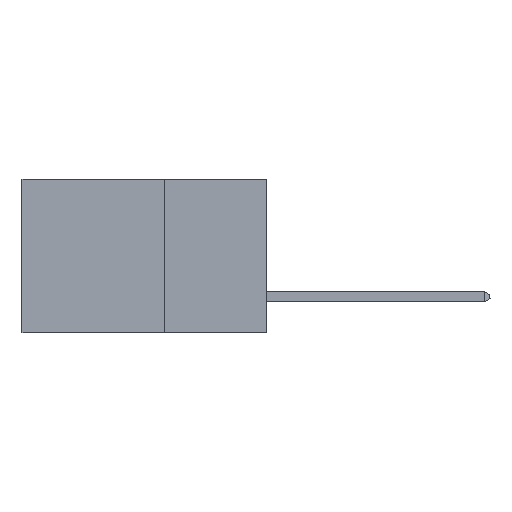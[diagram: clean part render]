
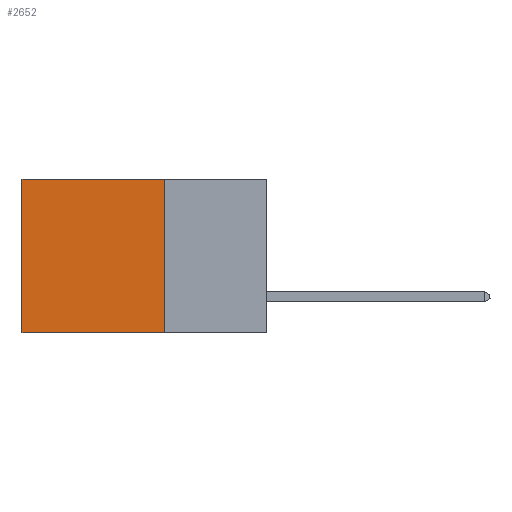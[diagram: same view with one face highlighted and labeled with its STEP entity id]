
A CAD part, left-side view. The second image highlights one B-rep face of the part: STEP entity #2652.
In plain terms, the highlighted planar face has unit normal (-1, 0, 0).
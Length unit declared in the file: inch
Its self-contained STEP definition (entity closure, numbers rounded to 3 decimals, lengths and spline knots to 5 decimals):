
#271 = CARTESIAN_POINT ( 'NONE',  ( 0.2875, 0.25, 0. ) ) ;
#722 = CARTESIAN_POINT ( 'NONE',  ( 0.2875, 0.25, -0.375 ) ) ;
#2652 = ADVANCED_FACE ( 'NONE', ( #4396 ), #6562, .F. ) ;
#2677 = VECTOR ( 'NONE', #5088, 39.37008 ) ;
#2813 = EDGE_CURVE ( 'NONE', #5606, #12103, #5889, .T. ) ;
#3095 = CARTESIAN_POINT ( 'NONE',  ( 0.2875, 0.25, -0.375 ) ) ;
#3446 = ORIENTED_EDGE ( 'NONE', *, *, #2813, .T. ) ;
#3755 = VECTOR ( 'NONE', #7795, 39.37008 ) ;
#3766 = ORIENTED_EDGE ( 'NONE', *, *, #13900, .F. ) ;
#4256 = CARTESIAN_POINT ( 'NONE',  ( 0.2875, 0.6, -0.375 ) ) ;
#4271 = VERTEX_POINT ( 'NONE', #7142 ) ;
#4396 = FACE_OUTER_BOUND ( 'NONE', #11799, .T. ) ;
#4600 = CARTESIAN_POINT ( 'NONE',  ( 0.2875, 0.25, -0.375 ) ) ;
#5088 = DIRECTION ( 'NONE',  ( 0., 1., 0. ) ) ;
#5606 = VERTEX_POINT ( 'NONE', #7146 ) ;
#5709 = LINE ( 'NONE', #12401, #6722 ) ;
#5889 = LINE ( 'NONE', #6635, #3755 ) ;
#5900 = LINE ( 'NONE', #4600, #6425 ) ;
#6425 = VECTOR ( 'NONE', #9101, 39.37008 ) ;
#6562 = PLANE ( 'NONE',  #11405 ) ;
#6635 = CARTESIAN_POINT ( 'NONE',  ( 0.2875, 0.6, -0.375 ) ) ;
#6722 = VECTOR ( 'NONE', #8974, 39.37008 ) ;
#6753 = EDGE_CURVE ( 'NONE', #11811, #5606, #5709, .T. ) ;
#7142 = CARTESIAN_POINT ( 'NONE',  ( 0.2875, 0.25, -0.375 ) ) ;
#7146 = CARTESIAN_POINT ( 'NONE',  ( 0.2875, 0.6, 0. ) ) ;
#7255 = LINE ( 'NONE', #722, #2677 ) ;
#7795 = DIRECTION ( 'NONE',  ( 0., 0., -1. ) ) ;
#8974 = DIRECTION ( 'NONE',  ( 0., 1., 0. ) ) ;
#9101 = DIRECTION ( 'NONE',  ( 0., 0., -1. ) ) ;
#9267 = EDGE_CURVE ( 'NONE', #4271, #12103, #7255, .T. ) ;
#9344 = ORIENTED_EDGE ( 'NONE', *, *, #9267, .F. ) ;
#11082 = ORIENTED_EDGE ( 'NONE', *, *, #6753, .T. ) ;
#11405 = AXIS2_PLACEMENT_3D ( 'NONE', #3095, #13044, #13256 ) ;
#11799 = EDGE_LOOP ( 'NONE', ( #3446, #9344, #3766, #11082 ) ) ;
#11811 = VERTEX_POINT ( 'NONE', #271 ) ;
#12103 = VERTEX_POINT ( 'NONE', #4256 ) ;
#12401 = CARTESIAN_POINT ( 'NONE',  ( 0.2875, 0.25, 0. ) ) ;
#13044 = DIRECTION ( 'NONE',  ( 1., 0., 0. ) ) ;
#13256 = DIRECTION ( 'NONE',  ( 0., 0., -1. ) ) ;
#13900 = EDGE_CURVE ( 'NONE', #11811, #4271, #5900, .T. ) ;
